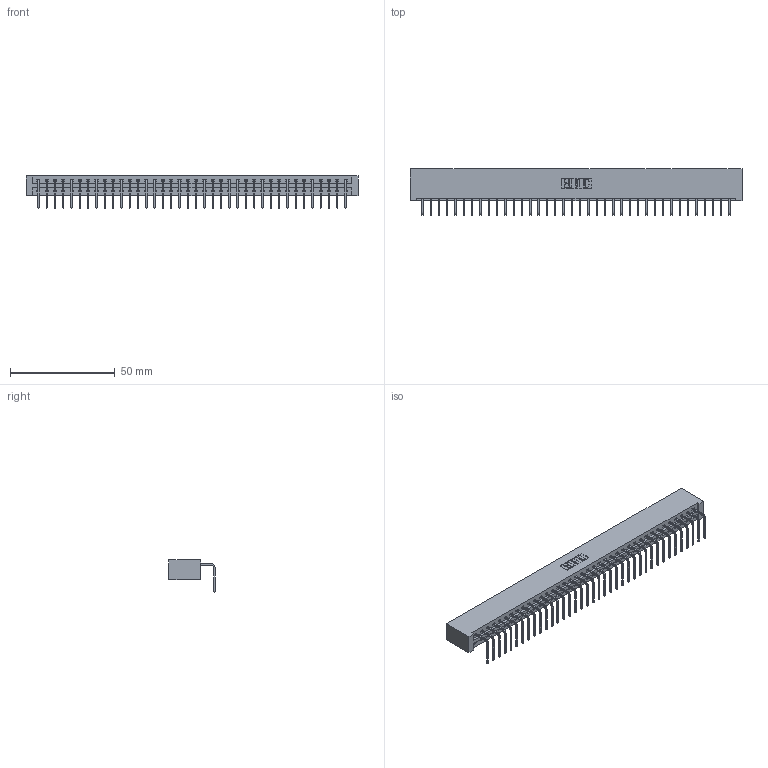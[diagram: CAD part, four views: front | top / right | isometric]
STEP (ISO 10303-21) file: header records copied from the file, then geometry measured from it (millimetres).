
FILE_DESCRIPTION (( 'STEP AP203' ), '1' );
FILE_NAME ('837-038-558-101.STEP', '2021-08-04T15:34:56', ( '' ), ( '' ), 'SwSTEP 2.0', 'SolidWorks 2020', '' );
FILE_SCHEMA (( 'CONFIG_CONTROL_DESIGN' ));
Length unit declared in the file: inch
Products named in the file (3): 837-038-558-101; 837 Part_No Mounting Lugs; 345-292-001_558 Tail - 2
Assembly tree (39 placements, depth 2):
  837-038-558-101
    837 Part_No Mounting Lugs
    345-292-001_558 Tail - 2  x38
Bounding box: 158.45 x 22.17 x 15.37 mm (x, y, z)
Volume: 17283 mm3; surface area: 18596.5 mm2
Topology: 39 solids, 39 shells, 2538 faces, 7659 edges, 5054 vertices
Faces by surface type: plane 1890, cylinder 648
Entity records: 28571 total; most frequent: CARTESIAN_POINT 4984, ORIENTED_EDGE 4958, DIRECTION 4195, EDGE_CURVE 2479, VECTOR 2359, LINE 2359, VERTEX_POINT 1650, AXIS2_PLACEMENT_3D 918
